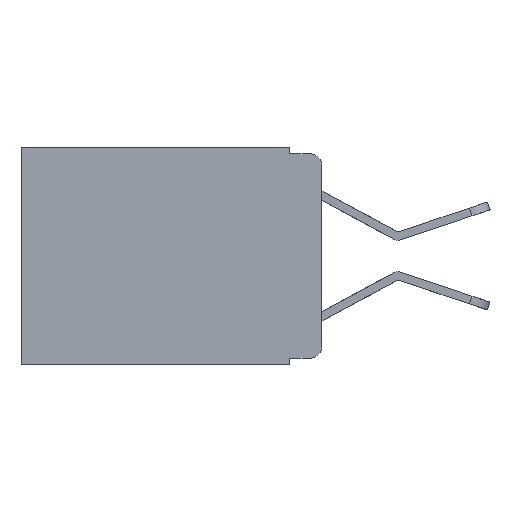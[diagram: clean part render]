
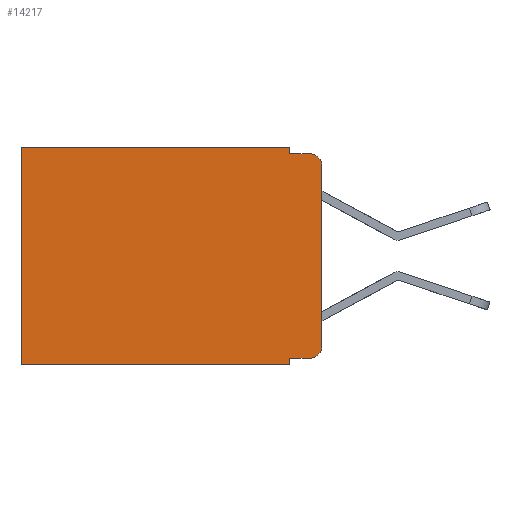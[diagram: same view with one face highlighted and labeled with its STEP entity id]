
A CAD part, left-side view. The second image highlights one B-rep face of the part: STEP entity #14217.
In plain terms, the highlighted planar face has unit normal (-1, 0, 0).
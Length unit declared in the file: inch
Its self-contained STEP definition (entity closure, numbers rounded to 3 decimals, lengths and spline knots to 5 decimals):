
#66 = LINE ( 'NONE', #12469, #4317 ) ;
#155 = CARTESIAN_POINT ( 'NONE',  ( 0.298, 0.473, 0. ) ) ;
#210 = DIRECTION ( 'NONE',  ( 0., -1., 0. ) ) ;
#379 = VERTEX_POINT ( 'NONE', #18676 ) ;
#395 = DIRECTION ( 'NONE',  ( 0., -1., 0. ) ) ;
#532 = ORIENTED_EDGE ( 'NONE', *, *, #19989, .T. ) ;
#1098 = VERTEX_POINT ( 'NONE', #5335 ) ;
#1520 = CARTESIAN_POINT ( 'NONE',  ( 0.298, 0.02, -0.01 ) ) ;
#1694 = VERTEX_POINT ( 'NONE', #8766 ) ;
#1925 = ORIENTED_EDGE ( 'NONE', *, *, #17437, .F. ) ;
#2250 = CARTESIAN_POINT ( 'NONE',  ( 0.298, 0.02, -0.313 ) ) ;
#2315 = VECTOR ( 'NONE', #210, 39.37008 ) ;
#2352 = CARTESIAN_POINT ( 'NONE',  ( 0.298, 0., 0. ) ) ;
#2354 = CARTESIAN_POINT ( 'NONE',  ( 0.298, 0., -0.343 ) ) ;
#2378 = PLANE ( 'NONE',  #5606 ) ;
#4075 = DIRECTION ( 'NONE',  ( 0., 0., -1. ) ) ;
#4159 = DIRECTION ( 'NONE',  ( 0., 0., -1. ) ) ;
#4161 = DIRECTION ( 'NONE',  ( 0., 1., 0. ) ) ;
#4317 = VECTOR ( 'NONE', #5333, 39.37008 ) ;
#4493 = LINE ( 'NONE', #2354, #13423 ) ;
#5022 = ORIENTED_EDGE ( 'NONE', *, *, #20298, .T. ) ;
#5097 = VECTOR ( 'NONE', #7734, 39.37008 ) ;
#5289 = ORIENTED_EDGE ( 'NONE', *, *, #9982, .F. ) ;
#5333 = DIRECTION ( 'NONE',  ( 0., 0., -1. ) ) ;
#5335 = CARTESIAN_POINT ( 'NONE',  ( 0.298, 0.473, -0.343 ) ) ;
#5606 = AXIS2_PLACEMENT_3D ( 'NONE', #16553, #6033, #18226 ) ;
#5890 = CARTESIAN_POINT ( 'NONE',  ( 0.298, 0.051, 0. ) ) ;
#6033 = DIRECTION ( 'NONE',  ( 1., 0., 0. ) ) ;
#6480 = VERTEX_POINT ( 'NONE', #11606 ) ;
#6490 = CARTESIAN_POINT ( 'NONE',  ( 0.298, 0.051, -0.333 ) ) ;
#6742 = CARTESIAN_POINT ( 'NONE',  ( 0.298, 0., -0.03 ) ) ;
#6973 = DIRECTION ( 'NONE',  ( 0., 0., -1. ) ) ;
#7174 = LINE ( 'NONE', #10986, #2315 ) ;
#7254 = EDGE_CURVE ( 'NONE', #1694, #7824, #7174, .T. ) ;
#7674 = CARTESIAN_POINT ( 'NONE',  ( 0.298, 0., -0.313 ) ) ;
#7734 = DIRECTION ( 'NONE',  ( 0., 0., -1. ) ) ;
#7824 = VERTEX_POINT ( 'NONE', #1520 ) ;
#8631 = DIRECTION ( 'NONE',  ( -1., 0., 0. ) ) ;
#8766 = CARTESIAN_POINT ( 'NONE',  ( 0.298, 0.051, -0.01 ) ) ;
#9040 = AXIS2_PLACEMENT_3D ( 'NONE', #18930, #8631, #20633 ) ;
#9982 = EDGE_CURVE ( 'NONE', #12712, #20308, #19417, .T. ) ;
#10986 = CARTESIAN_POINT ( 'NONE',  ( 0.298, 0.051, -0.01 ) ) ;
#11002 = EDGE_CURVE ( 'NONE', #12330, #1098, #66, .T. ) ;
#11008 = AXIS2_PLACEMENT_3D ( 'NONE', #2250, #14720, #4075 ) ;
#11236 = CARTESIAN_POINT ( 'NONE',  ( 0.298, 0.051, -0.333 ) ) ;
#11340 = EDGE_LOOP ( 'NONE', ( #5289, #532, #13130, #1925, #20413, #17484, #21572, #20923, #12103, #5022 ) ) ;
#11457 = CIRCLE ( 'NONE', #9040, 0.02 ) ;
#11606 = CARTESIAN_POINT ( 'NONE',  ( 0.298, 0.051, -0.343 ) ) ;
#11609 = DIRECTION ( 'NONE',  ( 0., 1., 0. ) ) ;
#11794 = FACE_OUTER_BOUND ( 'NONE', #11340, .T. ) ;
#12103 = ORIENTED_EDGE ( 'NONE', *, *, #21980, .T. ) ;
#12330 = VERTEX_POINT ( 'NONE', #155 ) ;
#12469 = CARTESIAN_POINT ( 'NONE',  ( 0.298, 0.473, 0. ) ) ;
#12712 = VERTEX_POINT ( 'NONE', #6742 ) ;
#13130 = ORIENTED_EDGE ( 'NONE', *, *, #7254, .F. ) ;
#13423 = VECTOR ( 'NONE', #4161, 39.37008 ) ;
#13973 = CARTESIAN_POINT ( 'NONE',  ( 0.298, 0.051, 0. ) ) ;
#13981 = LINE ( 'NONE', #5890, #5097 ) ;
#14117 = VECTOR ( 'NONE', #395, 39.37008 ) ;
#14217 = ADVANCED_FACE ( 'NONE', ( #11794 ), #2378, .F. ) ;
#14409 = VERTEX_POINT ( 'NONE', #6490 ) ;
#14597 = VERTEX_POINT ( 'NONE', #20866 ) ;
#14720 = DIRECTION ( 'NONE',  ( -1., 0., 0. ) ) ;
#14812 = EDGE_CURVE ( 'NONE', #14409, #6480, #22587, .T. ) ;
#15457 = LINE ( 'NONE', #21743, #20459 ) ;
#16553 = CARTESIAN_POINT ( 'NONE',  ( 0.298, 0., 0. ) ) ;
#17437 = EDGE_CURVE ( 'NONE', #14597, #1694, #13981, .T. ) ;
#17484 = ORIENTED_EDGE ( 'NONE', *, *, #11002, .T. ) ;
#17626 = VECTOR ( 'NONE', #6973, 39.37008 ) ;
#17897 = EDGE_CURVE ( 'NONE', #6480, #1098, #4493, .T. ) ;
#18226 = DIRECTION ( 'NONE',  ( 0., 0., -1. ) ) ;
#18676 = CARTESIAN_POINT ( 'NONE',  ( 0.298, 0.02, -0.333 ) ) ;
#18867 = VECTOR ( 'NONE', #4159, 39.37008 ) ;
#18930 = CARTESIAN_POINT ( 'NONE',  ( 0.298, 0.02, -0.03 ) ) ;
#19417 = LINE ( 'NONE', #2352, #18867 ) ;
#19457 = CIRCLE ( 'NONE', #11008, 0.02 ) ;
#19693 = LINE ( 'NONE', #11236, #14117 ) ;
#19989 = EDGE_CURVE ( 'NONE', #12712, #7824, #11457, .T. ) ;
#20298 = EDGE_CURVE ( 'NONE', #379, #20308, #19457, .T. ) ;
#20308 = VERTEX_POINT ( 'NONE', #7674 ) ;
#20413 = ORIENTED_EDGE ( 'NONE', *, *, #22113, .T. ) ;
#20459 = VECTOR ( 'NONE', #11609, 39.37008 ) ;
#20633 = DIRECTION ( 'NONE',  ( 0., 0., -1. ) ) ;
#20866 = CARTESIAN_POINT ( 'NONE',  ( 0.298, 0.051, 0. ) ) ;
#20923 = ORIENTED_EDGE ( 'NONE', *, *, #14812, .F. ) ;
#21572 = ORIENTED_EDGE ( 'NONE', *, *, #17897, .F. ) ;
#21743 = CARTESIAN_POINT ( 'NONE',  ( 0.298, 0., 0. ) ) ;
#21980 = EDGE_CURVE ( 'NONE', #14409, #379, #19693, .T. ) ;
#22113 = EDGE_CURVE ( 'NONE', #14597, #12330, #15457, .T. ) ;
#22587 = LINE ( 'NONE', #13973, #17626 ) ;
